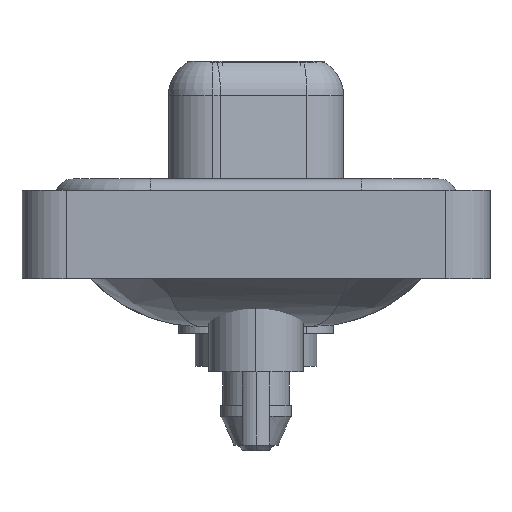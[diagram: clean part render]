
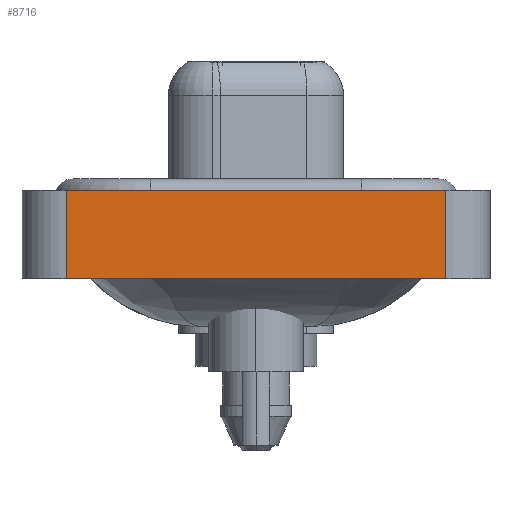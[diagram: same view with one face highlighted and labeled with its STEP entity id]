
A CAD part, left-side view. The second image highlights one B-rep face of the part: STEP entity #8716.
In plain terms, the highlighted planar face has unit normal (-1, 0, 0).
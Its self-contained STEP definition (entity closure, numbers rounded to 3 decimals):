
#1182 = CARTESIAN_POINT ( 'NONE',  ( -7.25, -8.55, -3.6 ) ) ;
#1275 = DIRECTION ( 'NONE',  ( 0., 0., 1. ) ) ;
#1457 = FACE_OUTER_BOUND ( 'NONE', #4106, .T. ) ;
#1577 = ORIENTED_EDGE ( 'NONE', *, *, #9117, .T. ) ;
#3487 = ORIENTED_EDGE ( 'NONE', *, *, #9063, .T. ) ;
#4106 = EDGE_LOOP ( 'NONE', ( #3487, #11322, #4623, #1577 ) ) ;
#4136 = PLANE ( 'NONE',  #5322 ) ;
#4623 = ORIENTED_EDGE ( 'NONE', *, *, #7959, .F. ) ;
#4763 = CARTESIAN_POINT ( 'NONE',  ( -7.25, -8.55, 0.4 ) ) ;
#5193 = DIRECTION ( 'NONE',  ( 0., -1., 0. ) ) ;
#5215 = VECTOR ( 'NONE', #11689, 1000. ) ;
#5267 = CARTESIAN_POINT ( 'NONE',  ( -7.25, -8.55, -3.6 ) ) ;
#5273 = LINE ( 'NONE', #6764, #14874 ) ;
#5322 = AXIS2_PLACEMENT_3D ( 'NONE', #9412, #13455, #8192 ) ;
#6513 = LINE ( 'NONE', #1182, #9265 ) ;
#6764 = CARTESIAN_POINT ( 'NONE',  ( -7.25, 8.55, -3.6 ) ) ;
#7959 = EDGE_CURVE ( 'NONE', #15347, #12739, #5273, .T. ) ;
#8192 = DIRECTION ( 'NONE',  ( 0., 0., 1. ) ) ;
#8716 = ADVANCED_FACE ( 'NONE', ( #1457 ), #4136, .T. ) ;
#9063 = EDGE_CURVE ( 'NONE', #11090, #16192, #11750, .T. ) ;
#9078 = LINE ( 'NONE', #4763, #5215 ) ;
#9117 = EDGE_CURVE ( 'NONE', #15347, #11090, #6513, .T. ) ;
#9265 = VECTOR ( 'NONE', #5193, 1000. ) ;
#9412 = CARTESIAN_POINT ( 'NONE',  ( -7.25, -8.55, -3.6 ) ) ;
#11090 = VERTEX_POINT ( 'NONE', #5267 ) ;
#11322 = ORIENTED_EDGE ( 'NONE', *, *, #11871, .F. ) ;
#11689 = DIRECTION ( 'NONE',  ( 0., -1., 0. ) ) ;
#11750 = LINE ( 'NONE', #17211, #16815 ) ;
#11871 = EDGE_CURVE ( 'NONE', #12739, #16192, #9078, .T. ) ;
#12739 = VERTEX_POINT ( 'NONE', #16924 ) ;
#13455 = DIRECTION ( 'NONE',  ( -1., 0., 0. ) ) ;
#13601 = CARTESIAN_POINT ( 'NONE',  ( -7.25, 8.55, -3.6 ) ) ;
#14851 = CARTESIAN_POINT ( 'NONE',  ( -7.25, -8.55, 0.4 ) ) ;
#14874 = VECTOR ( 'NONE', #1275, 1000. ) ;
#15347 = VERTEX_POINT ( 'NONE', #13601 ) ;
#15808 = DIRECTION ( 'NONE',  ( 0., 0., 1. ) ) ;
#16192 = VERTEX_POINT ( 'NONE', #14851 ) ;
#16815 = VECTOR ( 'NONE', #15808, 1000. ) ;
#16924 = CARTESIAN_POINT ( 'NONE',  ( -7.25, 8.55, 0.4 ) ) ;
#17211 = CARTESIAN_POINT ( 'NONE',  ( -7.25, -8.55, -3.6 ) ) ;
